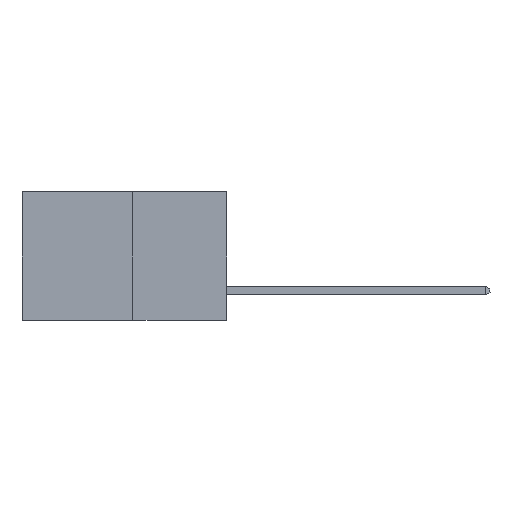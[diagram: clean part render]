
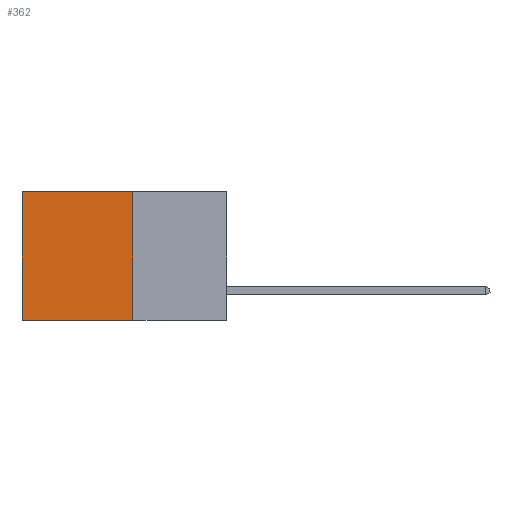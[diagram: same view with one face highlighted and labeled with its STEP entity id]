
A CAD part, left-side view. The second image highlights one B-rep face of the part: STEP entity #362.
In plain terms, the highlighted planar face has unit normal (-1, 0, 0).
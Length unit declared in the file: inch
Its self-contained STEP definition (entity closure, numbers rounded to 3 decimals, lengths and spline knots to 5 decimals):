
#42 = FACE_OUTER_BOUND ( 'NONE', #11834, .T. ) ;
#66 = CARTESIAN_POINT ( 'NONE',  ( 0.277, 0.27, -0.37 ) ) ;
#119 = ORIENTED_EDGE ( 'NONE', *, *, #1311, .T. ) ;
#362 = ADVANCED_FACE ( 'NONE', ( #42 ), #3846, .F. ) ;
#495 = CARTESIAN_POINT ( 'NONE',  ( 0.277, 0.27, 0. ) ) ;
#760 = LINE ( 'NONE', #8519, #9171 ) ;
#959 = VECTOR ( 'NONE', #3155, 39.37008 ) ;
#1226 = VERTEX_POINT ( 'NONE', #11801 ) ;
#1232 = CARTESIAN_POINT ( 'NONE',  ( 0.277, 0.59, -0.37 ) ) ;
#1311 = EDGE_CURVE ( 'NONE', #7559, #5742, #760, .T. ) ;
#1632 = DIRECTION ( 'NONE',  ( 0., 1., 0. ) ) ;
#1694 = EDGE_CURVE ( 'NONE', #5742, #6010, #3658, .T. ) ;
#2164 = DIRECTION ( 'NONE',  ( 0., 0., -1. ) ) ;
#2361 = CARTESIAN_POINT ( 'NONE',  ( 0.277, 0.59, -0.37 ) ) ;
#2667 = ORIENTED_EDGE ( 'NONE', *, *, #1694, .T. ) ;
#3122 = AXIS2_PLACEMENT_3D ( 'NONE', #11295, #3362, #7304 ) ;
#3155 = DIRECTION ( 'NONE',  ( 0., 0., -1. ) ) ;
#3362 = DIRECTION ( 'NONE',  ( 1., 0., 0. ) ) ;
#3658 = LINE ( 'NONE', #2361, #959 ) ;
#3846 = PLANE ( 'NONE',  #3122 ) ;
#5358 = CARTESIAN_POINT ( 'NONE',  ( 0.277, 0.59, 0. ) ) ;
#5742 = VERTEX_POINT ( 'NONE', #5358 ) ;
#5876 = ORIENTED_EDGE ( 'NONE', *, *, #11503, .F. ) ;
#6010 = VERTEX_POINT ( 'NONE', #1232 ) ;
#6783 = DIRECTION ( 'NONE',  ( 0., 1., 0. ) ) ;
#7038 = VECTOR ( 'NONE', #2164, 39.37008 ) ;
#7304 = DIRECTION ( 'NONE',  ( 0., 0., -1. ) ) ;
#7559 = VERTEX_POINT ( 'NONE', #495 ) ;
#8519 = CARTESIAN_POINT ( 'NONE',  ( 0.277, 0.27, 0. ) ) ;
#8554 = ORIENTED_EDGE ( 'NONE', *, *, #10191, .F. ) ;
#8831 = LINE ( 'NONE', #66, #11320 ) ;
#9171 = VECTOR ( 'NONE', #1632, 39.37008 ) ;
#9878 = LINE ( 'NONE', #13847, #7038 ) ;
#10191 = EDGE_CURVE ( 'NONE', #1226, #6010, #8831, .T. ) ;
#11295 = CARTESIAN_POINT ( 'NONE',  ( 0.277, 0.27, -0.37 ) ) ;
#11320 = VECTOR ( 'NONE', #6783, 39.37008 ) ;
#11503 = EDGE_CURVE ( 'NONE', #7559, #1226, #9878, .T. ) ;
#11801 = CARTESIAN_POINT ( 'NONE',  ( 0.277, 0.27, -0.37 ) ) ;
#11834 = EDGE_LOOP ( 'NONE', ( #2667, #8554, #5876, #119 ) ) ;
#13847 = CARTESIAN_POINT ( 'NONE',  ( 0.277, 0.27, -0.37 ) ) ;
